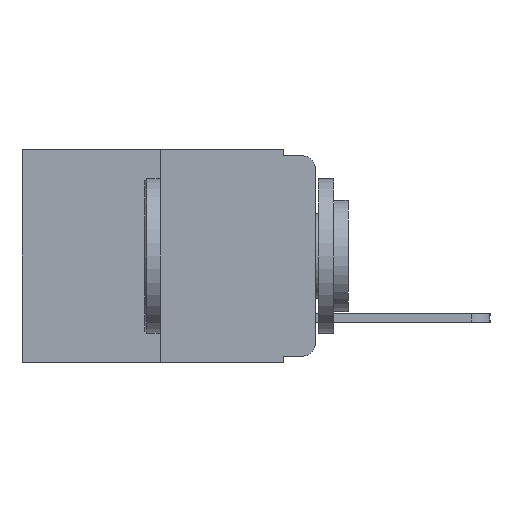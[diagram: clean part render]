
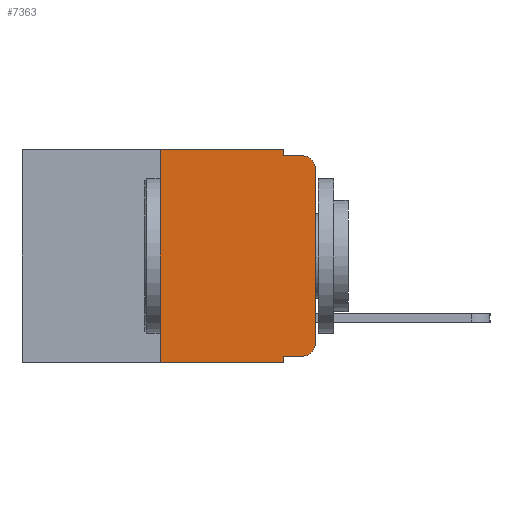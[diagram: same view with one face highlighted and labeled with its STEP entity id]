
A CAD part, left-side view. The second image highlights one B-rep face of the part: STEP entity #7363.
In plain terms, the highlighted planar face has unit normal (-1, 0, 0).
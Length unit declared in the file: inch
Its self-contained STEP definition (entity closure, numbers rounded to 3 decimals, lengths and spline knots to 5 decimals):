
#280 = VECTOR ( 'NONE', #6355, 39.37008 ) ;
#707 = CARTESIAN_POINT ( 'NONE',  ( 0., 0.02, -0.03 ) ) ;
#1176 = VERTEX_POINT ( 'NONE', #7221 ) ;
#1355 = CARTESIAN_POINT ( 'NONE',  ( 0., 0.051, 0. ) ) ;
#1558 = CARTESIAN_POINT ( 'NONE',  ( 0., 0.051, -0.333 ) ) ;
#1737 = CARTESIAN_POINT ( 'NONE',  ( 0., 0.051, -0.01 ) ) ;
#2427 = DIRECTION ( 'NONE',  ( 0., 0., -1. ) ) ;
#3368 = DIRECTION ( 'NONE',  ( 0., 0., 1. ) ) ;
#3401 = CARTESIAN_POINT ( 'NONE',  ( 0., 0.473, 0. ) ) ;
#3451 = DIRECTION ( 'NONE',  ( 0., -1., 0. ) ) ;
#3928 = ORIENTED_EDGE ( 'NONE', *, *, #8772, .F. ) ;
#4195 = CARTESIAN_POINT ( 'NONE',  ( 0., 0.25, -0.343 ) ) ;
#4251 = CARTESIAN_POINT ( 'NONE',  ( 0., 0.25, 0. ) ) ;
#4320 = EDGE_CURVE ( 'NONE', #18592, #5394, #11662, .T. ) ;
#4798 = DIRECTION ( 'NONE',  ( 0., -1., 0. ) ) ;
#4975 = ORIENTED_EDGE ( 'NONE', *, *, #14982, .T. ) ;
#5042 = CARTESIAN_POINT ( 'NONE',  ( 0., 0., 0. ) ) ;
#5279 = VERTEX_POINT ( 'NONE', #4195 ) ;
#5394 = VERTEX_POINT ( 'NONE', #7835 ) ;
#5456 = EDGE_CURVE ( 'NONE', #15903, #18592, #20959, .T. ) ;
#5696 = AXIS2_PLACEMENT_3D ( 'NONE', #707, #12385, #2427 ) ;
#5932 = DIRECTION ( 'NONE',  ( 0., 0., 1. ) ) ;
#6291 = LINE ( 'NONE', #1737, #10160 ) ;
#6355 = DIRECTION ( 'NONE',  ( 0., 0., -1. ) ) ;
#6583 = EDGE_CURVE ( 'NONE', #15903, #12850, #18403, .T. ) ;
#6609 = VERTEX_POINT ( 'NONE', #19463 ) ;
#7221 = CARTESIAN_POINT ( 'NONE',  ( 0., 0.051, 0. ) ) ;
#7318 = AXIS2_PLACEMENT_3D ( 'NONE', #3401, #10067, #21402 ) ;
#7363 = ADVANCED_FACE ( 'NONE', ( #19870 ), #19782, .F. ) ;
#7444 = VECTOR ( 'NONE', #3368, 39.37008 ) ;
#7672 = EDGE_CURVE ( 'NONE', #5279, #9521, #19111, .T. ) ;
#7767 = CIRCLE ( 'NONE', #5696, 0.02 ) ;
#7835 = CARTESIAN_POINT ( 'NONE',  ( 0., 0., -0.313 ) ) ;
#8376 = CARTESIAN_POINT ( 'NONE',  ( 0., 0.02, -0.313 ) ) ;
#8529 = EDGE_CURVE ( 'NONE', #9521, #1176, #20077, .T. ) ;
#8772 = EDGE_CURVE ( 'NONE', #1176, #6609, #15051, .T. ) ;
#8921 = CARTESIAN_POINT ( 'NONE',  ( 0., 0.051, -0.343 ) ) ;
#9022 = VECTOR ( 'NONE', #16129, 39.37008 ) ;
#9039 = CARTESIAN_POINT ( 'NONE',  ( 0., 0.25, 0. ) ) ;
#9072 = DIRECTION ( 'NONE',  ( 0., 0., -1. ) ) ;
#9383 = ORIENTED_EDGE ( 'NONE', *, *, #6583, .F. ) ;
#9521 = VERTEX_POINT ( 'NONE', #9039 ) ;
#9790 = EDGE_LOOP ( 'NONE', ( #11702, #20299, #16539, #3928, #12749, #13259, #4975, #9383, #14775, #10937 ) ) ;
#9886 = EDGE_CURVE ( 'NONE', #6609, #14339, #6291, .T. ) ;
#10027 = DIRECTION ( 'NONE',  ( 0., 0., -1. ) ) ;
#10067 = DIRECTION ( 'NONE',  ( 1., 0., 0. ) ) ;
#10160 = VECTOR ( 'NONE', #3451, 39.37008 ) ;
#10173 = VECTOR ( 'NONE', #9072, 39.37008 ) ;
#10937 = ORIENTED_EDGE ( 'NONE', *, *, #4320, .T. ) ;
#10995 = EDGE_CURVE ( 'NONE', #11085, #14339, #7767, .T. ) ;
#11085 = VERTEX_POINT ( 'NONE', #15771 ) ;
#11484 = VECTOR ( 'NONE', #4798, 39.37008 ) ;
#11662 = CIRCLE ( 'NONE', #18365, 0.02 ) ;
#11702 = ORIENTED_EDGE ( 'NONE', *, *, #12103, .T. ) ;
#12103 = EDGE_CURVE ( 'NONE', #5394, #11085, #16167, .T. ) ;
#12337 = CARTESIAN_POINT ( 'NONE',  ( 0., 0.051, 0. ) ) ;
#12385 = DIRECTION ( 'NONE',  ( -1., 0., 0. ) ) ;
#12749 = ORIENTED_EDGE ( 'NONE', *, *, #8529, .F. ) ;
#12850 = VERTEX_POINT ( 'NONE', #8921 ) ;
#13259 = ORIENTED_EDGE ( 'NONE', *, *, #7672, .F. ) ;
#14072 = DIRECTION ( 'NONE',  ( 0., -1., 0. ) ) ;
#14330 = VECTOR ( 'NONE', #5932, 39.37008 ) ;
#14339 = VERTEX_POINT ( 'NONE', #18355 ) ;
#14515 = CARTESIAN_POINT ( 'NONE',  ( 0., 0.051, -0.333 ) ) ;
#14775 = ORIENTED_EDGE ( 'NONE', *, *, #5456, .T. ) ;
#14982 = EDGE_CURVE ( 'NONE', #5279, #12850, #21181, .T. ) ;
#15051 = LINE ( 'NONE', #12337, #10173 ) ;
#15614 = CARTESIAN_POINT ( 'NONE',  ( 0., 0.473, -0.343 ) ) ;
#15771 = CARTESIAN_POINT ( 'NONE',  ( 0., 0., -0.03 ) ) ;
#15903 = VERTEX_POINT ( 'NONE', #1558 ) ;
#16129 = DIRECTION ( 'NONE',  ( 0., -1., 0. ) ) ;
#16167 = LINE ( 'NONE', #5042, #7444 ) ;
#16405 = VECTOR ( 'NONE', #14072, 39.37008 ) ;
#16539 = ORIENTED_EDGE ( 'NONE', *, *, #9886, .F. ) ;
#18355 = CARTESIAN_POINT ( 'NONE',  ( 0., 0.02, -0.01 ) ) ;
#18365 = AXIS2_PLACEMENT_3D ( 'NONE', #8376, #19749, #10027 ) ;
#18403 = LINE ( 'NONE', #1355, #280 ) ;
#18592 = VERTEX_POINT ( 'NONE', #19504 ) ;
#19111 = LINE ( 'NONE', #4251, #14330 ) ;
#19456 = CARTESIAN_POINT ( 'NONE',  ( 0., 0.473, 0. ) ) ;
#19463 = CARTESIAN_POINT ( 'NONE',  ( 0., 0.051, -0.01 ) ) ;
#19504 = CARTESIAN_POINT ( 'NONE',  ( 0., 0.02, -0.333 ) ) ;
#19749 = DIRECTION ( 'NONE',  ( -1., 0., 0. ) ) ;
#19782 = PLANE ( 'NONE',  #7318 ) ;
#19870 = FACE_OUTER_BOUND ( 'NONE', #9790, .T. ) ;
#20077 = LINE ( 'NONE', #19456, #11484 ) ;
#20299 = ORIENTED_EDGE ( 'NONE', *, *, #10995, .T. ) ;
#20959 = LINE ( 'NONE', #14515, #9022 ) ;
#21181 = LINE ( 'NONE', #15614, #16405 ) ;
#21402 = DIRECTION ( 'NONE',  ( 0., 0., -1. ) ) ;
